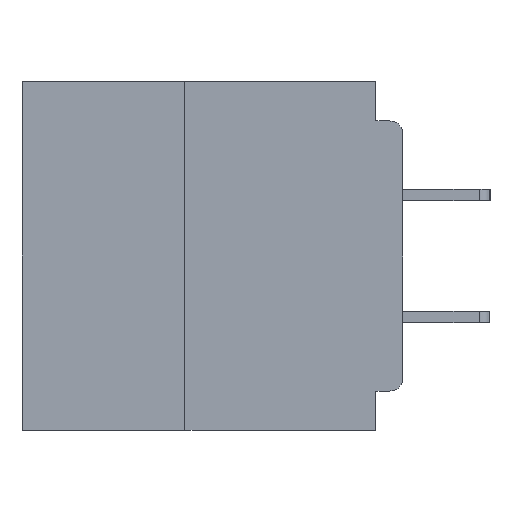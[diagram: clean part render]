
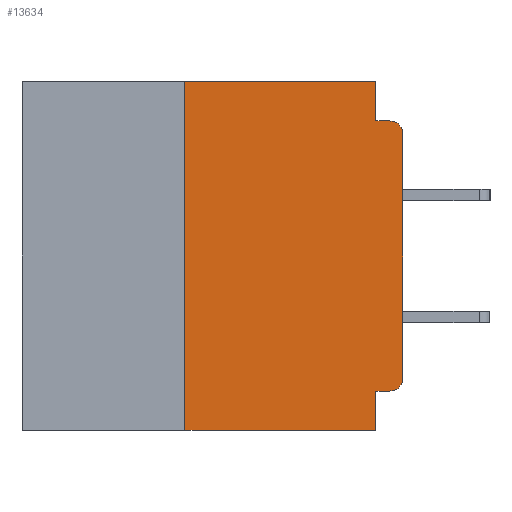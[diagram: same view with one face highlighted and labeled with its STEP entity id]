
A CAD part, left-side view. The second image highlights one B-rep face of the part: STEP entity #13634.
In plain terms, the highlighted planar face has unit normal (-1, 0, 0).
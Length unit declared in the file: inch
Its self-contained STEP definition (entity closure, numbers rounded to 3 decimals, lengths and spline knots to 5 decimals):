
#95 = VERTEX_POINT ( 'NONE', #13676 ) ;
#252 = DIRECTION ( 'NONE',  ( 0., -1., 0. ) ) ;
#575 = LINE ( 'NONE', #47227, #32971 ) ;
#602 = CARTESIAN_POINT ( 'NONE',  ( 0., 0.015, -0.355 ) ) ;
#1460 = ORIENTED_EDGE ( 'NONE', *, *, #4583, .F. ) ;
#1863 = AXIS2_PLACEMENT_3D ( 'NONE', #28622, #4241, #32616 ) ;
#2038 = ORIENTED_EDGE ( 'NONE', *, *, #48953, .F. ) ;
#2231 = VECTOR ( 'NONE', #42471, 39.37008 ) ;
#3024 = EDGE_CURVE ( 'NONE', #39947, #25699, #34582, .T. ) ;
#3354 = VERTEX_POINT ( 'NONE', #28486 ) ;
#3474 = CARTESIAN_POINT ( 'NONE',  ( 0., 0.25, -0.4 ) ) ;
#4241 = DIRECTION ( 'NONE',  ( -1., 0., 0. ) ) ;
#4466 = DIRECTION ( 'NONE',  ( 0., 1., 0. ) ) ;
#4583 = EDGE_CURVE ( 'NONE', #25373, #3354, #15581, .T. ) ;
#5346 = EDGE_LOOP ( 'NONE', ( #39284, #44431, #1460, #23140, #14747, #33120, #24161, #2038, #24112, #19984 ) ) ;
#5973 = CARTESIAN_POINT ( 'NONE',  ( 0., 0.031, 0. ) ) ;
#5976 = CARTESIAN_POINT ( 'NONE',  ( 0., 0.031, -0.4 ) ) ;
#6370 = VECTOR ( 'NONE', #35552, 39.37008 ) ;
#6397 = CARTESIAN_POINT ( 'NONE',  ( 0., 0.031, 0. ) ) ;
#6705 = VECTOR ( 'NONE', #22068, 39.37008 ) ;
#7883 = DIRECTION ( 'NONE',  ( 0., 0., -1. ) ) ;
#9142 = DIRECTION ( 'NONE',  ( -1., 0., 0. ) ) ;
#10119 = EDGE_CURVE ( 'NONE', #14620, #25373, #28407, .T. ) ;
#10332 = VERTEX_POINT ( 'NONE', #43790 ) ;
#10870 = DIRECTION ( 'NONE',  ( 0., 0., -1. ) ) ;
#13634 = ADVANCED_FACE ( 'NONE', ( #51224 ), #28204, .F. ) ;
#13676 = CARTESIAN_POINT ( 'NONE',  ( 0., 0.031, -0.355 ) ) ;
#14620 = VERTEX_POINT ( 'NONE', #6397 ) ;
#14747 = ORIENTED_EDGE ( 'NONE', *, *, #18117, .F. ) ;
#15343 = AXIS2_PLACEMENT_3D ( 'NONE', #33433, #9142, #37416 ) ;
#15581 = LINE ( 'NONE', #48851, #25143 ) ;
#16116 = EDGE_CURVE ( 'NONE', #19249, #49014, #39668, .T. ) ;
#18117 = EDGE_CURVE ( 'NONE', #10332, #14620, #45269, .T. ) ;
#18389 = CARTESIAN_POINT ( 'NONE',  ( 0., 0., 0. ) ) ;
#18716 = EDGE_CURVE ( 'NONE', #39175, #39947, #48339, .T. ) ;
#19249 = VERTEX_POINT ( 'NONE', #3474 ) ;
#19984 = ORIENTED_EDGE ( 'NONE', *, *, #18716, .T. ) ;
#20763 = DIRECTION ( 'NONE',  ( 0., -1., 0. ) ) ;
#21586 = EDGE_CURVE ( 'NONE', #19249, #10332, #28068, .T. ) ;
#22068 = DIRECTION ( 'NONE',  ( 0., 0., -1. ) ) ;
#22103 = CARTESIAN_POINT ( 'NONE',  ( 0., 0., -0.34 ) ) ;
#23140 = ORIENTED_EDGE ( 'NONE', *, *, #10119, .F. ) ;
#23456 = EDGE_CURVE ( 'NONE', #39175, #95, #49136, .T. ) ;
#24112 = ORIENTED_EDGE ( 'NONE', *, *, #23456, .F. ) ;
#24161 = ORIENTED_EDGE ( 'NONE', *, *, #16116, .T. ) ;
#25143 = VECTOR ( 'NONE', #20763, 39.37008 ) ;
#25373 = VERTEX_POINT ( 'NONE', #44928 ) ;
#25627 = AXIS2_PLACEMENT_3D ( 'NONE', #52157, #32207, #7883 ) ;
#25699 = VERTEX_POINT ( 'NONE', #47007 ) ;
#28068 = LINE ( 'NONE', #31564, #6370 ) ;
#28204 = PLANE ( 'NONE',  #25627 ) ;
#28407 = LINE ( 'NONE', #5973, #6705 ) ;
#28486 = CARTESIAN_POINT ( 'NONE',  ( 0., 0.015, -0.045 ) ) ;
#28622 = CARTESIAN_POINT ( 'NONE',  ( 0., 0.015, -0.34 ) ) ;
#28725 = CARTESIAN_POINT ( 'NONE',  ( 0., 0.437, -0.4 ) ) ;
#28856 = CARTESIAN_POINT ( 'NONE',  ( 0., 0., -0.355 ) ) ;
#29071 = VECTOR ( 'NONE', #252, 39.37008 ) ;
#31564 = CARTESIAN_POINT ( 'NONE',  ( 0., 0.25, -0.4 ) ) ;
#32207 = DIRECTION ( 'NONE',  ( 1., 0., 0. ) ) ;
#32616 = DIRECTION ( 'NONE',  ( 0., 0., -1. ) ) ;
#32971 = VECTOR ( 'NONE', #10870, 39.37008 ) ;
#33120 = ORIENTED_EDGE ( 'NONE', *, *, #21586, .F. ) ;
#33433 = CARTESIAN_POINT ( 'NONE',  ( 0., 0.015, -0.06 ) ) ;
#34582 = LINE ( 'NONE', #18389, #2231 ) ;
#34583 = VECTOR ( 'NONE', #44759, 39.37008 ) ;
#35387 = EDGE_CURVE ( 'NONE', #25699, #3354, #51121, .T. ) ;
#35552 = DIRECTION ( 'NONE',  ( 0., 0., 1. ) ) ;
#36676 = CARTESIAN_POINT ( 'NONE',  ( 0., 0.437, 0. ) ) ;
#37416 = DIRECTION ( 'NONE',  ( 0., 0., -1. ) ) ;
#39175 = VERTEX_POINT ( 'NONE', #602 ) ;
#39284 = ORIENTED_EDGE ( 'NONE', *, *, #3024, .T. ) ;
#39668 = LINE ( 'NONE', #28725, #29071 ) ;
#39947 = VERTEX_POINT ( 'NONE', #22103 ) ;
#42471 = DIRECTION ( 'NONE',  ( 0., 0., 1. ) ) ;
#43790 = CARTESIAN_POINT ( 'NONE',  ( 0., 0.25, 0. ) ) ;
#44431 = ORIENTED_EDGE ( 'NONE', *, *, #35387, .T. ) ;
#44759 = DIRECTION ( 'NONE',  ( 0., -1., 0. ) ) ;
#44928 = CARTESIAN_POINT ( 'NONE',  ( 0., 0.031, -0.045 ) ) ;
#45269 = LINE ( 'NONE', #36676, #34583 ) ;
#47007 = CARTESIAN_POINT ( 'NONE',  ( 0., 0., -0.06 ) ) ;
#47227 = CARTESIAN_POINT ( 'NONE',  ( 0., 0.031, -0.4 ) ) ;
#47892 = VECTOR ( 'NONE', #4466, 39.37008 ) ;
#48339 = CIRCLE ( 'NONE', #1863, 0.015 ) ;
#48851 = CARTESIAN_POINT ( 'NONE',  ( 0., 0., -0.045 ) ) ;
#48953 = EDGE_CURVE ( 'NONE', #95, #49014, #575, .T. ) ;
#49014 = VERTEX_POINT ( 'NONE', #5976 ) ;
#49136 = LINE ( 'NONE', #28856, #47892 ) ;
#51121 = CIRCLE ( 'NONE', #15343, 0.015 ) ;
#51224 = FACE_OUTER_BOUND ( 'NONE', #5346, .T. ) ;
#52157 = CARTESIAN_POINT ( 'NONE',  ( 0., 0.437, 0. ) ) ;
